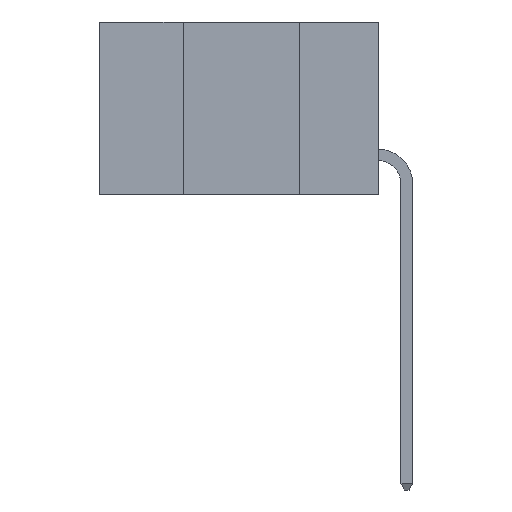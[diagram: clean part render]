
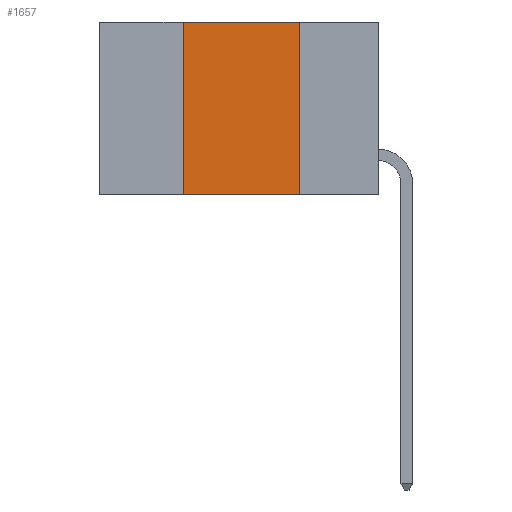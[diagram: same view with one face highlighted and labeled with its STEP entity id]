
A CAD part, left-side view. The second image highlights one B-rep face of the part: STEP entity #1657.
In plain terms, the highlighted planar face has unit normal (-1, 0, 0).
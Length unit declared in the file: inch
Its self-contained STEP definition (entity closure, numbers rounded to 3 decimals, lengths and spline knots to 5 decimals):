
#4 = CARTESIAN_POINT ( 'NONE',  ( 0., 0.6, -0.37 ) ) ;
#440 = CARTESIAN_POINT ( 'NONE',  ( 0., 0.6, 0. ) ) ;
#721 = ORIENTED_EDGE ( 'NONE', *, *, #8058, .T. ) ;
#925 = LINE ( 'NONE', #5747, #7331 ) ;
#1657 = ADVANCED_FACE ( 'NONE', ( #1960 ), #10757, .F. ) ;
#1717 = DIRECTION ( 'NONE',  ( 0., -1., 0. ) ) ;
#1844 = DIRECTION ( 'NONE',  ( 0., -1., 0. ) ) ;
#1960 = FACE_OUTER_BOUND ( 'NONE', #9609, .T. ) ;
#2176 = LINE ( 'NONE', #6180, #8938 ) ;
#2472 = VERTEX_POINT ( 'NONE', #10829 ) ;
#2982 = ORIENTED_EDGE ( 'NONE', *, *, #10203, .F. ) ;
#3102 = CARTESIAN_POINT ( 'NONE',  ( 0., 0.17, -0.37 ) ) ;
#3376 = VECTOR ( 'NONE', #1717, 39.37008 ) ;
#3633 = LINE ( 'NONE', #4368, #7779 ) ;
#4130 = DIRECTION ( 'NONE',  ( 0., 0., -1. ) ) ;
#4308 = DIRECTION ( 'NONE',  ( 0., 0., 1. ) ) ;
#4368 = CARTESIAN_POINT ( 'NONE',  ( 0., 0.42, -0.37 ) ) ;
#5519 = CARTESIAN_POINT ( 'NONE',  ( 0., 0.42, 0. ) ) ;
#5747 = CARTESIAN_POINT ( 'NONE',  ( 0., 0.17, -0.37 ) ) ;
#6180 = CARTESIAN_POINT ( 'NONE',  ( 0., 0.6, 0. ) ) ;
#6414 = VERTEX_POINT ( 'NONE', #5519 ) ;
#6560 = VERTEX_POINT ( 'NONE', #3102 ) ;
#6908 = AXIS2_PLACEMENT_3D ( 'NONE', #440, #10147, #9588 ) ;
#7061 = VERTEX_POINT ( 'NONE', #10542 ) ;
#7331 = VECTOR ( 'NONE', #4130, 39.37008 ) ;
#7421 = ORIENTED_EDGE ( 'NONE', *, *, #9166, .F. ) ;
#7777 = LINE ( 'NONE', #4, #3376 ) ;
#7779 = VECTOR ( 'NONE', #4308, 39.37008 ) ;
#8058 = EDGE_CURVE ( 'NONE', #2472, #6560, #7777, .T. ) ;
#8620 = EDGE_CURVE ( 'NONE', #2472, #6414, #3633, .T. ) ;
#8938 = VECTOR ( 'NONE', #1844, 39.37008 ) ;
#9166 = EDGE_CURVE ( 'NONE', #6414, #7061, #2176, .T. ) ;
#9588 = DIRECTION ( 'NONE',  ( 0., 0., -1. ) ) ;
#9589 = ORIENTED_EDGE ( 'NONE', *, *, #8620, .F. ) ;
#9609 = EDGE_LOOP ( 'NONE', ( #2982, #7421, #9589, #721 ) ) ;
#10147 = DIRECTION ( 'NONE',  ( 1., 0., 0. ) ) ;
#10203 = EDGE_CURVE ( 'NONE', #7061, #6560, #925, .T. ) ;
#10542 = CARTESIAN_POINT ( 'NONE',  ( 0., 0.17, 0. ) ) ;
#10757 = PLANE ( 'NONE',  #6908 ) ;
#10829 = CARTESIAN_POINT ( 'NONE',  ( 0., 0.42, -0.37 ) ) ;
